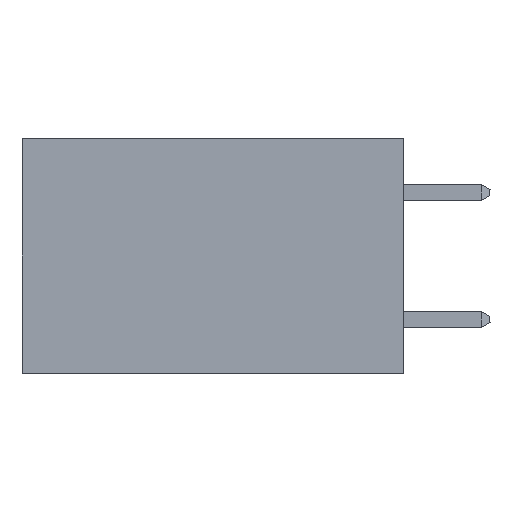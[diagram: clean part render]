
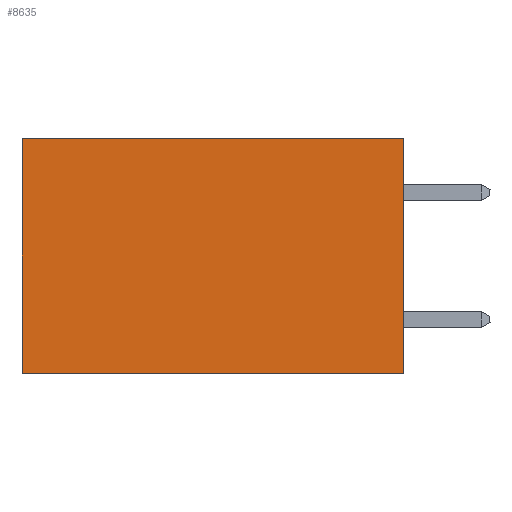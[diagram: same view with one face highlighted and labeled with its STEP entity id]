
A CAD part, left-side view. The second image highlights one B-rep face of the part: STEP entity #8635.
In plain terms, the highlighted planar face has unit normal (-1, 0, 0).
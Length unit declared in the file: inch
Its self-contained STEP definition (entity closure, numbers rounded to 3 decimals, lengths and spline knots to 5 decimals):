
#206 = DIRECTION ( 'NONE',  ( 0., 0., -1. ) ) ;
#378 = LINE ( 'NONE', #11475, #26955 ) ;
#1720 = LINE ( 'NONE', #29796, #24688 ) ;
#2821 = DIRECTION ( 'NONE',  ( 1., 0., 0. ) ) ;
#4018 = AXIS2_PLACEMENT_3D ( 'NONE', #15632, #2821, #206 ) ;
#5421 = VERTEX_POINT ( 'NONE', #29304 ) ;
#6280 = ORIENTED_EDGE ( 'NONE', *, *, #20810, .F. ) ;
#6521 = LINE ( 'NONE', #25376, #28199 ) ;
#7131 = ORIENTED_EDGE ( 'NONE', *, *, #10042, .F. ) ;
#8635 = ADVANCED_FACE ( 'NONE', ( #20444 ), #18325, .F. ) ;
#9039 = CARTESIAN_POINT ( 'NONE',  ( 0.2875, 0., -0.37 ) ) ;
#9187 = ORIENTED_EDGE ( 'NONE', *, *, #15010, .T. ) ;
#10042 = EDGE_CURVE ( 'NONE', #26589, #28158, #23165, .T. ) ;
#10899 = CARTESIAN_POINT ( 'NONE',  ( 0.2875, 0., 0. ) ) ;
#11475 = CARTESIAN_POINT ( 'NONE',  ( 0.2875, 0., 0. ) ) ;
#12691 = EDGE_CURVE ( 'NONE', #5421, #28158, #1720, .T. ) ;
#12782 = EDGE_LOOP ( 'NONE', ( #21007, #7131, #6280, #9187 ) ) ;
#15010 = EDGE_CURVE ( 'NONE', #20492, #5421, #378, .T. ) ;
#15632 = CARTESIAN_POINT ( 'NONE',  ( 0.2875, 0., 0. ) ) ;
#18325 = PLANE ( 'NONE',  #4018 ) ;
#19319 = CARTESIAN_POINT ( 'NONE',  ( 0.2875, 0., -0.37 ) ) ;
#20444 = FACE_OUTER_BOUND ( 'NONE', #12782, .T. ) ;
#20492 = VERTEX_POINT ( 'NONE', #10899 ) ;
#20810 = EDGE_CURVE ( 'NONE', #20492, #26589, #6521, .T. ) ;
#21007 = ORIENTED_EDGE ( 'NONE', *, *, #12691, .T. ) ;
#22133 = DIRECTION ( 'NONE',  ( 0., 1., 0. ) ) ;
#22312 = DIRECTION ( 'NONE',  ( 0., 0., -1. ) ) ;
#23165 = LINE ( 'NONE', #19319, #32429 ) ;
#23190 = CARTESIAN_POINT ( 'NONE',  ( 0.2875, 0.6, -0.37 ) ) ;
#24688 = VECTOR ( 'NONE', #22312, 39.37008 ) ;
#25376 = CARTESIAN_POINT ( 'NONE',  ( 0.2875, 0., 0. ) ) ;
#26589 = VERTEX_POINT ( 'NONE', #9039 ) ;
#26871 = DIRECTION ( 'NONE',  ( 0., 1., 0. ) ) ;
#26955 = VECTOR ( 'NONE', #22133, 39.37008 ) ;
#28158 = VERTEX_POINT ( 'NONE', #23190 ) ;
#28199 = VECTOR ( 'NONE', #30392, 39.37008 ) ;
#29304 = CARTESIAN_POINT ( 'NONE',  ( 0.2875, 0.6, 0. ) ) ;
#29796 = CARTESIAN_POINT ( 'NONE',  ( 0.2875, 0.6, 0. ) ) ;
#30392 = DIRECTION ( 'NONE',  ( 0., 0., -1. ) ) ;
#32429 = VECTOR ( 'NONE', #26871, 39.37008 ) ;
